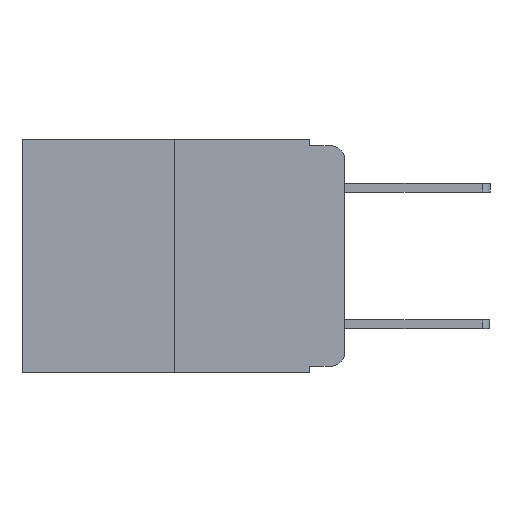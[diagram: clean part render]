
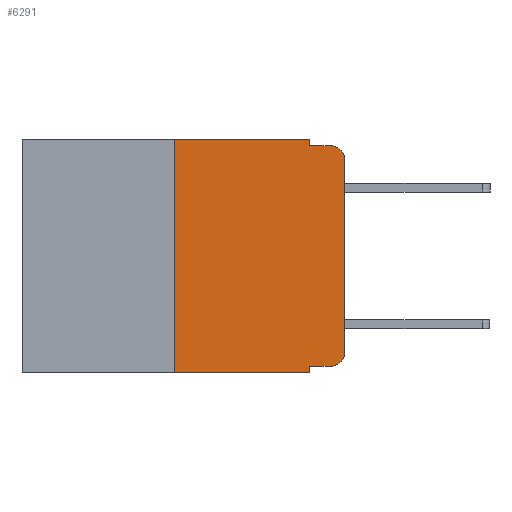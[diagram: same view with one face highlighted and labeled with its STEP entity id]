
A CAD part, left-side view. The second image highlights one B-rep face of the part: STEP entity #6291.
In plain terms, the highlighted planar face has unit normal (-1, 0, 0).
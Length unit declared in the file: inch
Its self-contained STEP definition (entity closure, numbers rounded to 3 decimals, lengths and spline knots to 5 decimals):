
#819 = VERTEX_POINT ( 'NONE', #13689 ) ;
#1022 = LINE ( 'NONE', #3237, #3781 ) ;
#1080 = CARTESIAN_POINT ( 'NONE',  ( 0., 0.473, 0. ) ) ;
#2008 = VERTEX_POINT ( 'NONE', #6410 ) ;
#2341 = ORIENTED_EDGE ( 'NONE', *, *, #8744, .T. ) ;
#2408 = VERTEX_POINT ( 'NONE', #3816 ) ;
#2555 = ORIENTED_EDGE ( 'NONE', *, *, #6494, .T. ) ;
#2575 = VERTEX_POINT ( 'NONE', #12664 ) ;
#2576 = EDGE_CURVE ( 'NONE', #10603, #2575, #3865, .T. ) ;
#2591 = VECTOR ( 'NONE', #7051, 39.37008 ) ;
#2659 = ORIENTED_EDGE ( 'NONE', *, *, #5742, .F. ) ;
#2948 = ORIENTED_EDGE ( 'NONE', *, *, #2576, .F. ) ;
#3057 = ORIENTED_EDGE ( 'NONE', *, *, #13307, .F. ) ;
#3237 = CARTESIAN_POINT ( 'NONE',  ( 0., 0.051, 0. ) ) ;
#3269 = ORIENTED_EDGE ( 'NONE', *, *, #13906, .F. ) ;
#3405 = DIRECTION ( 'NONE',  ( -1., 0., 0. ) ) ;
#3485 = ORIENTED_EDGE ( 'NONE', *, *, #6693, .T. ) ;
#3563 = ORIENTED_EDGE ( 'NONE', *, *, #13200, .F. ) ;
#3597 = ORIENTED_EDGE ( 'NONE', *, *, #12505, .T. ) ;
#3625 = ORIENTED_EDGE ( 'NONE', *, *, #10394, .T. ) ;
#3781 = VECTOR ( 'NONE', #8911, 39.37008 ) ;
#3785 = CARTESIAN_POINT ( 'NONE',  ( 0., 0.25, -0.343 ) ) ;
#3816 = CARTESIAN_POINT ( 'NONE',  ( 0., 0.02, -0.01 ) ) ;
#3865 = LINE ( 'NONE', #10513, #11941 ) ;
#3956 = VECTOR ( 'NONE', #10027, 39.37008 ) ;
#4022 = DIRECTION ( 'NONE',  ( 0., 0., -1. ) ) ;
#4100 = LINE ( 'NONE', #11706, #9992 ) ;
#4101 = VERTEX_POINT ( 'NONE', #3785 ) ;
#4109 = CARTESIAN_POINT ( 'NONE',  ( 0., 0.051, -0.01 ) ) ;
#4148 = PLANE ( 'NONE',  #9662 ) ;
#5418 = CARTESIAN_POINT ( 'NONE',  ( 0., 0., -0.03 ) ) ;
#5566 = CIRCLE ( 'NONE', #7970, 0.02 ) ;
#5742 = EDGE_CURVE ( 'NONE', #2575, #2408, #6818, .T. ) ;
#6095 = FACE_OUTER_BOUND ( 'NONE', #9616, .T. ) ;
#6291 = ADVANCED_FACE ( 'NONE', ( #6095 ), #4148, .F. ) ;
#6410 = CARTESIAN_POINT ( 'NONE',  ( 0., 0.25, 0. ) ) ;
#6447 = DIRECTION ( 'NONE',  ( 0., 0., -1. ) ) ;
#6494 = EDGE_CURVE ( 'NONE', #11015, #2408, #5566, .T. ) ;
#6526 = VERTEX_POINT ( 'NONE', #12252 ) ;
#6659 = DIRECTION ( 'NONE',  ( 0., -1., 0. ) ) ;
#6693 = EDGE_CURVE ( 'NONE', #4101, #13753, #11162, .T. ) ;
#6694 = CARTESIAN_POINT ( 'NONE',  ( 0., 0.02, -0.313 ) ) ;
#6766 = CARTESIAN_POINT ( 'NONE',  ( 0., 0.25, 0. ) ) ;
#6818 = LINE ( 'NONE', #4109, #9376 ) ;
#7051 = DIRECTION ( 'NONE',  ( 0., -1., 0. ) ) ;
#7541 = DIRECTION ( 'NONE',  ( 0., -1., 0. ) ) ;
#7794 = CARTESIAN_POINT ( 'NONE',  ( 0., 0.051, -0.333 ) ) ;
#7817 = DIRECTION ( 'NONE',  ( 0., 0., -1. ) ) ;
#7970 = AXIS2_PLACEMENT_3D ( 'NONE', #10087, #3405, #11163 ) ;
#8723 = CARTESIAN_POINT ( 'NONE',  ( 0., 0.051, -0.343 ) ) ;
#8744 = EDGE_CURVE ( 'NONE', #819, #11015, #4100, .T. ) ;
#8911 = DIRECTION ( 'NONE',  ( 0., 0., -1. ) ) ;
#9315 = CIRCLE ( 'NONE', #10688, 0.02 ) ;
#9376 = VECTOR ( 'NONE', #7541, 39.37008 ) ;
#9543 = LINE ( 'NONE', #6766, #3956 ) ;
#9616 = EDGE_LOOP ( 'NONE', ( #2341, #2555, #2659, #2948, #3057, #3269, #3485, #3563, #3597, #3625 ) ) ;
#9662 = AXIS2_PLACEMENT_3D ( 'NONE', #11817, #12854, #6447 ) ;
#9992 = VECTOR ( 'NONE', #12743, 39.37008 ) ;
#10027 = DIRECTION ( 'NONE',  ( 0., 0., 1. ) ) ;
#10087 = CARTESIAN_POINT ( 'NONE',  ( 0., 0.02, -0.03 ) ) ;
#10239 = LINE ( 'NONE', #13045, #13032 ) ;
#10394 = EDGE_CURVE ( 'NONE', #6526, #819, #9315, .T. ) ;
#10513 = CARTESIAN_POINT ( 'NONE',  ( 0., 0.051, 0. ) ) ;
#10603 = VERTEX_POINT ( 'NONE', #13488 ) ;
#10688 = AXIS2_PLACEMENT_3D ( 'NONE', #6694, #14136, #7817 ) ;
#11015 = VERTEX_POINT ( 'NONE', #5418 ) ;
#11104 = VERTEX_POINT ( 'NONE', #7794 ) ;
#11162 = LINE ( 'NONE', #13405, #2591 ) ;
#11163 = DIRECTION ( 'NONE',  ( 0., 0., -1. ) ) ;
#11212 = LINE ( 'NONE', #1080, #13669 ) ;
#11706 = CARTESIAN_POINT ( 'NONE',  ( 0., 0., 0. ) ) ;
#11817 = CARTESIAN_POINT ( 'NONE',  ( 0., 0.473, 0. ) ) ;
#11941 = VECTOR ( 'NONE', #4022, 39.37008 ) ;
#12252 = CARTESIAN_POINT ( 'NONE',  ( 0., 0.02, -0.333 ) ) ;
#12505 = EDGE_CURVE ( 'NONE', #11104, #6526, #10239, .T. ) ;
#12664 = CARTESIAN_POINT ( 'NONE',  ( 0., 0.051, -0.01 ) ) ;
#12743 = DIRECTION ( 'NONE',  ( 0., 0., 1. ) ) ;
#12854 = DIRECTION ( 'NONE',  ( 1., 0., 0. ) ) ;
#13032 = VECTOR ( 'NONE', #6659, 39.37008 ) ;
#13045 = CARTESIAN_POINT ( 'NONE',  ( 0., 0.051, -0.333 ) ) ;
#13200 = EDGE_CURVE ( 'NONE', #11104, #13753, #1022, .T. ) ;
#13307 = EDGE_CURVE ( 'NONE', #2008, #10603, #11212, .T. ) ;
#13405 = CARTESIAN_POINT ( 'NONE',  ( 0., 0.473, -0.343 ) ) ;
#13488 = CARTESIAN_POINT ( 'NONE',  ( 0., 0.051, 0. ) ) ;
#13669 = VECTOR ( 'NONE', #14308, 39.37008 ) ;
#13689 = CARTESIAN_POINT ( 'NONE',  ( 0., 0., -0.313 ) ) ;
#13753 = VERTEX_POINT ( 'NONE', #8723 ) ;
#13906 = EDGE_CURVE ( 'NONE', #4101, #2008, #9543, .T. ) ;
#14136 = DIRECTION ( 'NONE',  ( -1., 0., 0. ) ) ;
#14308 = DIRECTION ( 'NONE',  ( 0., -1., 0. ) ) ;
